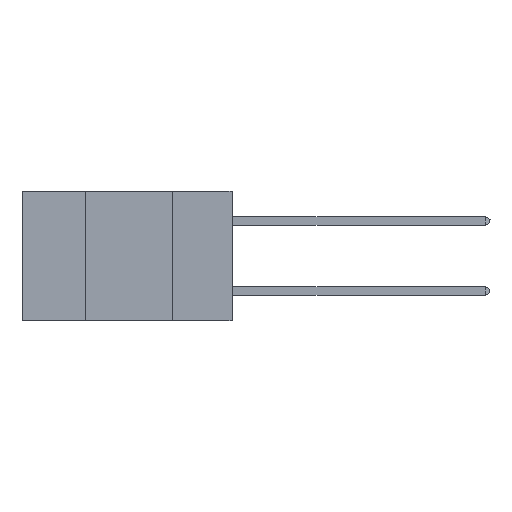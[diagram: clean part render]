
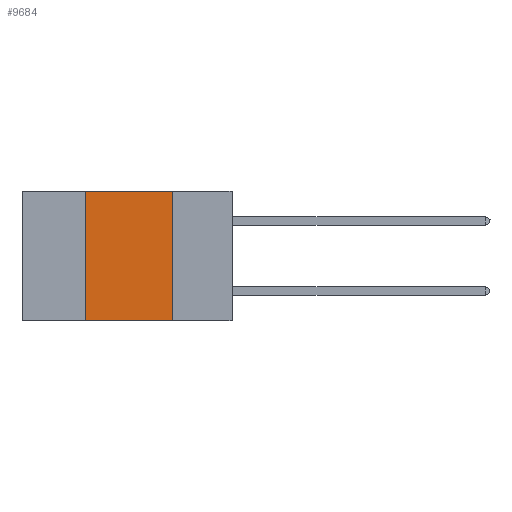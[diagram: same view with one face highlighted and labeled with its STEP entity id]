
A CAD part, left-side view. The second image highlights one B-rep face of the part: STEP entity #9684.
In plain terms, the highlighted planar face has unit normal (-1, 0, 0).
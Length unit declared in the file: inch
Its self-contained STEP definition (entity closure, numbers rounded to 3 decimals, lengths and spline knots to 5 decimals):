
#1224 = VECTOR ( 'NONE', #2261, 39.37008 ) ;
#1318 = VERTEX_POINT ( 'NONE', #14504 ) ;
#1349 = ORIENTED_EDGE ( 'NONE', *, *, #10105, .F. ) ;
#1364 = CARTESIAN_POINT ( 'NONE',  ( 0., 0.42, 0. ) ) ;
#1630 = DIRECTION ( 'NONE',  ( 0., 0., -1. ) ) ;
#1694 = VERTEX_POINT ( 'NONE', #1364 ) ;
#1852 = LINE ( 'NONE', #13237, #15459 ) ;
#1885 = LINE ( 'NONE', #3325, #14302 ) ;
#1974 = DIRECTION ( 'NONE',  ( 0., 0., 1. ) ) ;
#2011 = DIRECTION ( 'NONE',  ( 0., 0., -1. ) ) ;
#2261 = DIRECTION ( 'NONE',  ( 0., -1., 0. ) ) ;
#3325 = CARTESIAN_POINT ( 'NONE',  ( 0., 0.42, 0. ) ) ;
#3368 = LINE ( 'NONE', #13898, #11309 ) ;
#4152 = VERTEX_POINT ( 'NONE', #5925 ) ;
#5593 = VERTEX_POINT ( 'NONE', #15262 ) ;
#5671 = DIRECTION ( 'NONE',  ( 0., -1., 0. ) ) ;
#5778 = DIRECTION ( 'NONE',  ( 1., 0., 0. ) ) ;
#5925 = CARTESIAN_POINT ( 'NONE',  ( 0., 0.17, -0.37 ) ) ;
#6621 = ORIENTED_EDGE ( 'NONE', *, *, #7441, .F. ) ;
#7021 = PLANE ( 'NONE',  #10592 ) ;
#7111 = FACE_OUTER_BOUND ( 'NONE', #9272, .T. ) ;
#7434 = ORIENTED_EDGE ( 'NONE', *, *, #14200, .F. ) ;
#7441 = EDGE_CURVE ( 'NONE', #1318, #4152, #3368, .T. ) ;
#8753 = LINE ( 'NONE', #16238, #1224 ) ;
#9272 = EDGE_LOOP ( 'NONE', ( #6621, #1349, #7434, #10889 ) ) ;
#9684 = ADVANCED_FACE ( 'NONE', ( #7111 ), #7021, .F. ) ;
#10105 = EDGE_CURVE ( 'NONE', #1694, #1318, #1852, .T. ) ;
#10592 = AXIS2_PLACEMENT_3D ( 'NONE', #12162, #5778, #1630 ) ;
#10889 = ORIENTED_EDGE ( 'NONE', *, *, #11745, .T. ) ;
#11309 = VECTOR ( 'NONE', #2011, 39.37008 ) ;
#11745 = EDGE_CURVE ( 'NONE', #5593, #4152, #8753, .T. ) ;
#12162 = CARTESIAN_POINT ( 'NONE',  ( 0., 0.6, 0. ) ) ;
#13237 = CARTESIAN_POINT ( 'NONE',  ( 0., 0.6, 0. ) ) ;
#13898 = CARTESIAN_POINT ( 'NONE',  ( 0., 0.17, 0. ) ) ;
#14200 = EDGE_CURVE ( 'NONE', #5593, #1694, #1885, .T. ) ;
#14302 = VECTOR ( 'NONE', #1974, 39.37008 ) ;
#14504 = CARTESIAN_POINT ( 'NONE',  ( 0., 0.17, 0. ) ) ;
#15262 = CARTESIAN_POINT ( 'NONE',  ( 0., 0.42, -0.37 ) ) ;
#15459 = VECTOR ( 'NONE', #5671, 39.37008 ) ;
#16238 = CARTESIAN_POINT ( 'NONE',  ( 0., 0.6, -0.37 ) ) ;
